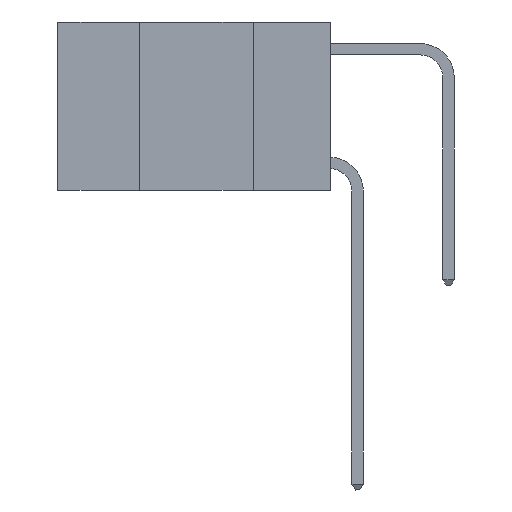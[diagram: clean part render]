
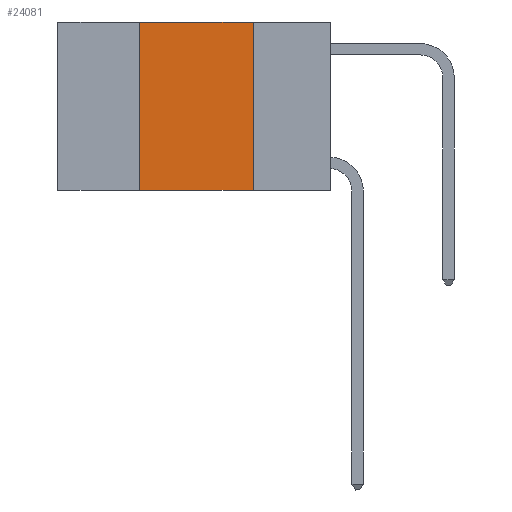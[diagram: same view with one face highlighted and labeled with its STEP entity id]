
A CAD part, left-side view. The second image highlights one B-rep face of the part: STEP entity #24081.
In plain terms, the highlighted planar face has unit normal (-1, 0, 0).
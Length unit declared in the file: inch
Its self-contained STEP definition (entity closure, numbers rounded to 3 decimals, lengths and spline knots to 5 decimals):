
#200 = EDGE_CURVE ( 'NONE', #18824, #23356, #18752, .T. ) ;
#1055 = CARTESIAN_POINT ( 'NONE',  ( 0., 0.6, 0. ) ) ;
#1589 = EDGE_CURVE ( 'NONE', #9201, #18824, #25262, .T. ) ;
#1648 = VERTEX_POINT ( 'NONE', #12602 ) ;
#2443 = PLANE ( 'NONE',  #10549 ) ;
#3527 = ORIENTED_EDGE ( 'NONE', *, *, #11474, .F. ) ;
#4711 = DIRECTION ( 'NONE',  ( 0., 0., -1. ) ) ;
#5989 = ORIENTED_EDGE ( 'NONE', *, *, #1589, .F. ) ;
#6863 = VECTOR ( 'NONE', #12289, 39.37008 ) ;
#9201 = VERTEX_POINT ( 'NONE', #18555 ) ;
#9391 = FACE_OUTER_BOUND ( 'NONE', #22206, .T. ) ;
#10184 = DIRECTION ( 'NONE',  ( 0., 0., 1. ) ) ;
#10549 = AXIS2_PLACEMENT_3D ( 'NONE', #15798, #18145, #4711 ) ;
#11474 = EDGE_CURVE ( 'NONE', #23356, #1648, #18435, .T. ) ;
#12090 = CARTESIAN_POINT ( 'NONE',  ( 0., 0.42, 0. ) ) ;
#12289 = DIRECTION ( 'NONE',  ( 0., -1., 0. ) ) ;
#12602 = CARTESIAN_POINT ( 'NONE',  ( 0., 0.17, -0.37 ) ) ;
#13175 = VECTOR ( 'NONE', #26276, 39.37008 ) ;
#15206 = CARTESIAN_POINT ( 'NONE',  ( 0., 0.17, 0. ) ) ;
#15798 = CARTESIAN_POINT ( 'NONE',  ( 0., 0.6, 0. ) ) ;
#17486 = ORIENTED_EDGE ( 'NONE', *, *, #23459, .T. ) ;
#18082 = CARTESIAN_POINT ( 'NONE',  ( 0., 0.17, 0. ) ) ;
#18145 = DIRECTION ( 'NONE',  ( 1., 0., 0. ) ) ;
#18435 = LINE ( 'NONE', #15206, #13175 ) ;
#18555 = CARTESIAN_POINT ( 'NONE',  ( 0., 0.42, -0.37 ) ) ;
#18601 = ORIENTED_EDGE ( 'NONE', *, *, #200, .F. ) ;
#18752 = LINE ( 'NONE', #1055, #6863 ) ;
#18824 = VERTEX_POINT ( 'NONE', #12090 ) ;
#19353 = VECTOR ( 'NONE', #10184, 39.37008 ) ;
#19536 = VECTOR ( 'NONE', #22802, 39.37008 ) ;
#20587 = CARTESIAN_POINT ( 'NONE',  ( 0., 0.6, -0.37 ) ) ;
#21258 = CARTESIAN_POINT ( 'NONE',  ( 0., 0.42, 0. ) ) ;
#22206 = EDGE_LOOP ( 'NONE', ( #3527, #18601, #5989, #17486 ) ) ;
#22802 = DIRECTION ( 'NONE',  ( 0., -1., 0. ) ) ;
#23356 = VERTEX_POINT ( 'NONE', #18082 ) ;
#23459 = EDGE_CURVE ( 'NONE', #9201, #1648, #25448, .T. ) ;
#24081 = ADVANCED_FACE ( 'NONE', ( #9391 ), #2443, .F. ) ;
#25262 = LINE ( 'NONE', #21258, #19353 ) ;
#25448 = LINE ( 'NONE', #20587, #19536 ) ;
#26276 = DIRECTION ( 'NONE',  ( 0., 0., -1. ) ) ;
